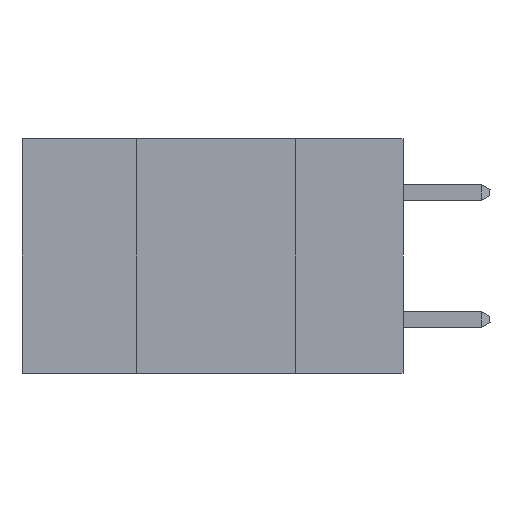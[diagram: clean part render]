
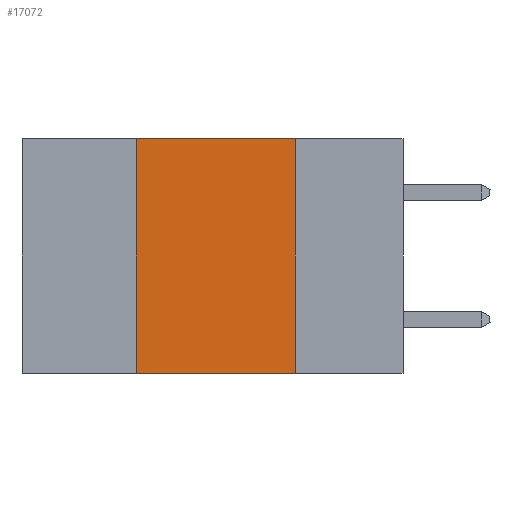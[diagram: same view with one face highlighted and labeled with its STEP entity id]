
A CAD part, left-side view. The second image highlights one B-rep face of the part: STEP entity #17072.
In plain terms, the highlighted planar face has unit normal (-1, 0, 0).
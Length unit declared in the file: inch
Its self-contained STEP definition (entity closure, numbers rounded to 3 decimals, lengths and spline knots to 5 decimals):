
#2229 = CARTESIAN_POINT ( 'NONE',  ( 0., 0.42, 0. ) ) ;
#3241 = PLANE ( 'NONE',  #24662 ) ;
#3672 = CARTESIAN_POINT ( 'NONE',  ( 0., 0.17, 0. ) ) ;
#5301 = DIRECTION ( 'NONE',  ( 0., 0., 1. ) ) ;
#6215 = LINE ( 'NONE', #2229, #26581 ) ;
#6909 = EDGE_CURVE ( 'NONE', #19660, #18743, #27580, .T. ) ;
#7080 = DIRECTION ( 'NONE',  ( 0., -1., 0. ) ) ;
#7648 = CARTESIAN_POINT ( 'NONE',  ( 0., 0.6, -0.37 ) ) ;
#9269 = VERTEX_POINT ( 'NONE', #29754 ) ;
#10491 = VECTOR ( 'NONE', #7080, 39.37008 ) ;
#10644 = FACE_OUTER_BOUND ( 'NONE', #39207, .T. ) ;
#10962 = LINE ( 'NONE', #7648, #28327 ) ;
#12803 = EDGE_CURVE ( 'NONE', #32440, #18743, #10962, .T. ) ;
#16909 = ORIENTED_EDGE ( 'NONE', *, *, #12803, .T. ) ;
#17072 = ADVANCED_FACE ( 'NONE', ( #10644 ), #3241, .F. ) ;
#17998 = CARTESIAN_POINT ( 'NONE',  ( 0., 0.42, -0.37 ) ) ;
#18725 = ORIENTED_EDGE ( 'NONE', *, *, #26670, .F. ) ;
#18743 = VERTEX_POINT ( 'NONE', #40096 ) ;
#19128 = ORIENTED_EDGE ( 'NONE', *, *, #6909, .F. ) ;
#19660 = VERTEX_POINT ( 'NONE', #37285 ) ;
#24662 = AXIS2_PLACEMENT_3D ( 'NONE', #29185, #28861, #25784 ) ;
#25784 = DIRECTION ( 'NONE',  ( 0., 0., -1. ) ) ;
#26321 = DIRECTION ( 'NONE',  ( 0., -1., 0. ) ) ;
#26581 = VECTOR ( 'NONE', #5301, 39.37008 ) ;
#26670 = EDGE_CURVE ( 'NONE', #32440, #9269, #6215, .T. ) ;
#27580 = LINE ( 'NONE', #3672, #32791 ) ;
#28327 = VECTOR ( 'NONE', #26321, 39.37008 ) ;
#28861 = DIRECTION ( 'NONE',  ( 1., 0., 0. ) ) ;
#29185 = CARTESIAN_POINT ( 'NONE',  ( 0., 0.6, 0. ) ) ;
#29646 = CARTESIAN_POINT ( 'NONE',  ( 0., 0.6, 0. ) ) ;
#29754 = CARTESIAN_POINT ( 'NONE',  ( 0., 0.42, 0. ) ) ;
#30799 = ORIENTED_EDGE ( 'NONE', *, *, #46371, .F. ) ;
#32440 = VERTEX_POINT ( 'NONE', #17998 ) ;
#32791 = VECTOR ( 'NONE', #38990, 39.37008 ) ;
#36638 = LINE ( 'NONE', #29646, #10491 ) ;
#37285 = CARTESIAN_POINT ( 'NONE',  ( 0., 0.17, 0. ) ) ;
#38990 = DIRECTION ( 'NONE',  ( 0., 0., -1. ) ) ;
#39207 = EDGE_LOOP ( 'NONE', ( #19128, #30799, #18725, #16909 ) ) ;
#40096 = CARTESIAN_POINT ( 'NONE',  ( 0., 0.17, -0.37 ) ) ;
#46371 = EDGE_CURVE ( 'NONE', #9269, #19660, #36638, .T. ) ;
